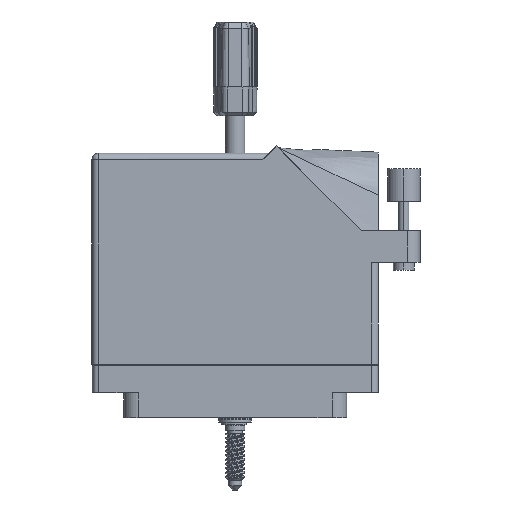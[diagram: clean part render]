
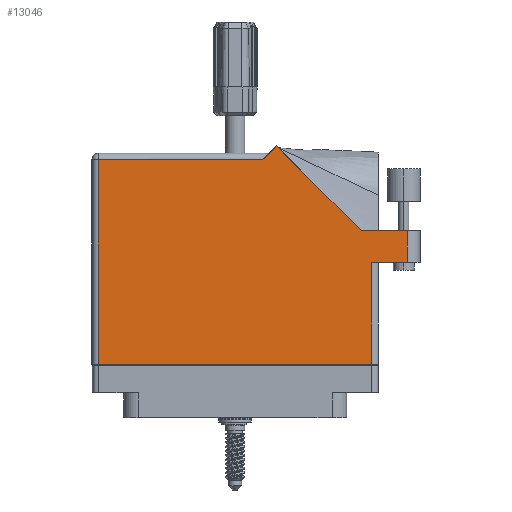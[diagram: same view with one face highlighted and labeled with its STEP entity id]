
A CAD part, front view. The second image highlights one B-rep face of the part: STEP entity #13046.
In plain terms, the highlighted face is planar.
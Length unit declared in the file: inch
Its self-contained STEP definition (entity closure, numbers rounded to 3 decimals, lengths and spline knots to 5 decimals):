
#228 = VERTEX_POINT ( 'NONE', #1435 ) ;
#423 = DIRECTION ( 'NONE',  ( 1., 0., 0. ) ) ;
#1435 = CARTESIAN_POINT ( 'NONE',  ( 1.3155, 0.88, 0.765 ) ) ;
#1860 = LINE ( 'NONE', #49390, #16212 ) ;
#4561 = ORIENTED_EDGE ( 'NONE', *, *, #57773, .T. ) ;
#5267 = VERTEX_POINT ( 'NONE', #40942 ) ;
#6207 = EDGE_CURVE ( 'NONE', #81607, #34487, #99181, .T. ) ;
#6785 = ORIENTED_EDGE ( 'NONE', *, *, #78815, .T. ) ;
#12689 = LINE ( 'NONE', #36624, #35468 ) ;
#13046 = ADVANCED_FACE ( 'NONE', ( #67788 ), #31313, .F. ) ;
#13383 = LINE ( 'NONE', #29055, #66118 ) ;
#14155 = VERTEX_POINT ( 'NONE', #67922 ) ;
#16212 = VECTOR ( 'NONE', #95046, 39.37008 ) ;
#17645 = EDGE_LOOP ( 'NONE', ( #48962, #72528, #75848, #61518, #4561, #60042, #6785, #58085, #55096 ) ) ;
#20297 = VECTOR ( 'NONE', #84853, 39.37008 ) ;
#20437 = CARTESIAN_POINT ( 'NONE',  ( 1.3155, -0.1, 0.765 ) ) ;
#26051 = VECTOR ( 'NONE', #95370, 39.37008 ) ;
#27083 = DIRECTION ( 'NONE',  ( 0., -1., 0. ) ) ;
#27839 = VERTEX_POINT ( 'NONE', #52451 ) ;
#29055 = CARTESIAN_POINT ( 'NONE',  ( 1.3155, 0.88, 0.765 ) ) ;
#31313 = PLANE ( 'NONE',  #62778 ) ;
#31942 = CARTESIAN_POINT ( 'NONE',  ( 1.6525, 1.187, 0.765 ) ) ;
#31966 = LINE ( 'NONE', #93128, #49869 ) ;
#33434 = CARTESIAN_POINT ( 'NONE',  ( -1.3155, -0.1, 0.765 ) ) ;
#33988 = VERTEX_POINT ( 'NONE', #20437 ) ;
#34403 = CARTESIAN_POINT ( 'NONE',  ( 1.6525, 1.187, 0.765 ) ) ;
#34487 = VERTEX_POINT ( 'NONE', #52364 ) ;
#35468 = VECTOR ( 'NONE', #50955, 39.37008 ) ;
#36624 = CARTESIAN_POINT ( 'NONE',  ( 1.21192, 1.187, 0.765 ) ) ;
#37687 = VERTEX_POINT ( 'NONE', #33434 ) ;
#38352 = CARTESIAN_POINT ( 'NONE',  ( -1.3775, 1.93, 0.765 ) ) ;
#40440 = VECTOR ( 'NONE', #68281, 39.37008 ) ;
#40942 = CARTESIAN_POINT ( 'NONE',  ( 0.39821, 2.00071, 0.765 ) ) ;
#42364 = EDGE_CURVE ( 'NONE', #37687, #33988, #31966, .T. ) ;
#45168 = CARTESIAN_POINT ( 'NONE',  ( 0.3275, 1.93, 0.765 ) ) ;
#45754 = EDGE_CURVE ( 'NONE', #33988, #228, #13383, .T. ) ;
#48962 = ORIENTED_EDGE ( 'NONE', *, *, #95964, .T. ) ;
#49390 = CARTESIAN_POINT ( 'NONE',  ( 1.7775, 1.187, 0.765 ) ) ;
#49869 = VECTOR ( 'NONE', #92489, 39.37008 ) ;
#50955 = DIRECTION ( 'NONE',  ( -0.707, 0.707, 0. ) ) ;
#52364 = CARTESIAN_POINT ( 'NONE',  ( -1.3155, 1.868, 0.765 ) ) ;
#52451 = CARTESIAN_POINT ( 'NONE',  ( 1.6525, 0.88, 0.765 ) ) ;
#54365 = DIRECTION ( 'NONE',  ( 0., 0., -1. ) ) ;
#55096 = ORIENTED_EDGE ( 'NONE', *, *, #45754, .T. ) ;
#57773 = EDGE_CURVE ( 'NONE', #5267, #81607, #63230, .T. ) ;
#58085 = ORIENTED_EDGE ( 'NONE', *, *, #42364, .T. ) ;
#58399 = EDGE_CURVE ( 'NONE', #27839, #66668, #81441, .T. ) ;
#60042 = ORIENTED_EDGE ( 'NONE', *, *, #6207, .T. ) ;
#61518 = ORIENTED_EDGE ( 'NONE', *, *, #88206, .T. ) ;
#62778 = AXIS2_PLACEMENT_3D ( 'NONE', #38352, #54365, #69425 ) ;
#63230 = LINE ( 'NONE', #45168, #40440 ) ;
#63918 = LINE ( 'NONE', #89383, #67468 ) ;
#64482 = CARTESIAN_POINT ( 'NONE',  ( -1.3775, 1.868, 0.765 ) ) ;
#65890 = DIRECTION ( 'NONE',  ( 0., 1., 0. ) ) ;
#66118 = VECTOR ( 'NONE', #65890, 39.37008 ) ;
#66668 = VERTEX_POINT ( 'NONE', #34403 ) ;
#67468 = VECTOR ( 'NONE', #27083, 39.37008 ) ;
#67788 = FACE_OUTER_BOUND ( 'NONE', #17645, .T. ) ;
#67922 = CARTESIAN_POINT ( 'NONE',  ( 1.21192, 1.187, 0.765 ) ) ;
#68281 = DIRECTION ( 'NONE',  ( -0.707, -0.707, 0. ) ) ;
#68839 = VECTOR ( 'NONE', #423, 39.37008 ) ;
#68935 = LINE ( 'NONE', #75758, #68839 ) ;
#69425 = DIRECTION ( 'NONE',  ( -1., 0., 0. ) ) ;
#72528 = ORIENTED_EDGE ( 'NONE', *, *, #58399, .T. ) ;
#73008 = CARTESIAN_POINT ( 'NONE',  ( 0.2655, 1.868, 0.765 ) ) ;
#75758 = CARTESIAN_POINT ( 'NONE',  ( 1.3775, 0.88, 0.765 ) ) ;
#75848 = ORIENTED_EDGE ( 'NONE', *, *, #79824, .T. ) ;
#78815 = EDGE_CURVE ( 'NONE', #34487, #37687, #63918, .T. ) ;
#79824 = EDGE_CURVE ( 'NONE', #66668, #14155, #1860, .T. ) ;
#81441 = LINE ( 'NONE', #31942, #20297 ) ;
#81607 = VERTEX_POINT ( 'NONE', #73008 ) ;
#84853 = DIRECTION ( 'NONE',  ( 0., 1., 0. ) ) ;
#88206 = EDGE_CURVE ( 'NONE', #14155, #5267, #12689, .T. ) ;
#89383 = CARTESIAN_POINT ( 'NONE',  ( -1.3155, -0.1, 0.765 ) ) ;
#92489 = DIRECTION ( 'NONE',  ( 1., 0., 0. ) ) ;
#93128 = CARTESIAN_POINT ( 'NONE',  ( -1.3775, -0.1, 0.765 ) ) ;
#95046 = DIRECTION ( 'NONE',  ( -1., 0., 0. ) ) ;
#95370 = DIRECTION ( 'NONE',  ( -1., 0., 0. ) ) ;
#95964 = EDGE_CURVE ( 'NONE', #228, #27839, #68935, .T. ) ;
#99181 = LINE ( 'NONE', #64482, #26051 ) ;
